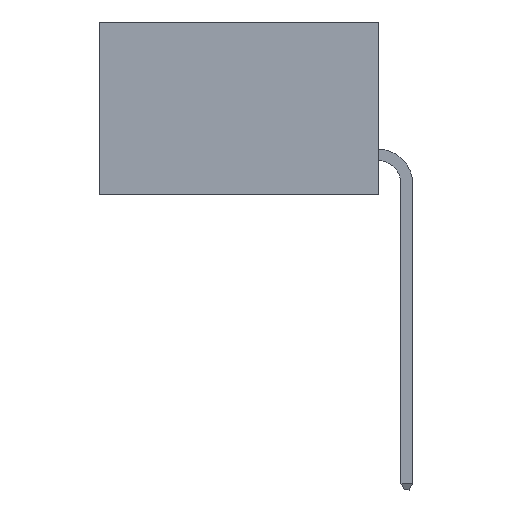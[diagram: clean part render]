
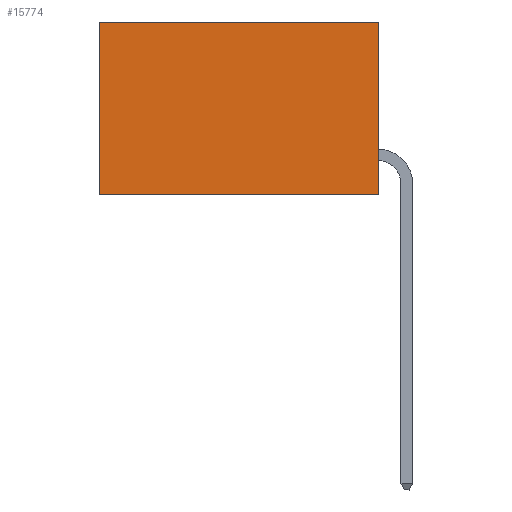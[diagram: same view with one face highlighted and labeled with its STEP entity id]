
A CAD part, left-side view. The second image highlights one B-rep face of the part: STEP entity #15774.
In plain terms, the highlighted planar face has unit normal (-1, 0, 0).
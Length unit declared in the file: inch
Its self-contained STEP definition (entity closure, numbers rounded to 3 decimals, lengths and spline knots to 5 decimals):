
#78 = ORIENTED_EDGE ( 'NONE', *, *, #14140, .T. ) ;
#652 = CARTESIAN_POINT ( 'NONE',  ( 0.298, 0., 0. ) ) ;
#923 = ORIENTED_EDGE ( 'NONE', *, *, #11105, .F. ) ;
#1417 = VERTEX_POINT ( 'NONE', #21766 ) ;
#1817 = LINE ( 'NONE', #8845, #7195 ) ;
#3545 = PLANE ( 'NONE',  #12620 ) ;
#3612 = VERTEX_POINT ( 'NONE', #7756 ) ;
#3830 = VECTOR ( 'NONE', #17193, 39.37008 ) ;
#5278 = ORIENTED_EDGE ( 'NONE', *, *, #18916, .F. ) ;
#5939 = EDGE_LOOP ( 'NONE', ( #15491, #5278, #923, #78 ) ) ;
#6220 = VECTOR ( 'NONE', #10168, 39.37008 ) ;
#6861 = LINE ( 'NONE', #8173, #6220 ) ;
#7195 = VECTOR ( 'NONE', #18887, 39.37008 ) ;
#7619 = DIRECTION ( 'NONE',  ( 1., 0., 0. ) ) ;
#7756 = CARTESIAN_POINT ( 'NONE',  ( 0.298, 0., -0.37 ) ) ;
#8173 = CARTESIAN_POINT ( 'NONE',  ( 0.298, 0.6, 0. ) ) ;
#8714 = VECTOR ( 'NONE', #22568, 39.37008 ) ;
#8845 = CARTESIAN_POINT ( 'NONE',  ( 0.298, 0., -0.37 ) ) ;
#9205 = LINE ( 'NONE', #19108, #3830 ) ;
#10168 = DIRECTION ( 'NONE',  ( 0., 0., -1. ) ) ;
#10492 = FACE_OUTER_BOUND ( 'NONE', #5939, .T. ) ;
#11105 = EDGE_CURVE ( 'NONE', #11674, #3612, #9205, .T. ) ;
#11674 = VERTEX_POINT ( 'NONE', #652 ) ;
#12620 = AXIS2_PLACEMENT_3D ( 'NONE', #25580, #7619, #21693 ) ;
#14073 = LINE ( 'NONE', #20533, #8714 ) ;
#14140 = EDGE_CURVE ( 'NONE', #11674, #1417, #14073, .T. ) ;
#15414 = CARTESIAN_POINT ( 'NONE',  ( 0.298, 0.6, -0.37 ) ) ;
#15491 = ORIENTED_EDGE ( 'NONE', *, *, #20212, .T. ) ;
#15774 = ADVANCED_FACE ( 'NONE', ( #10492 ), #3545, .F. ) ;
#17193 = DIRECTION ( 'NONE',  ( 0., 0., -1. ) ) ;
#18887 = DIRECTION ( 'NONE',  ( 0., 1., 0. ) ) ;
#18916 = EDGE_CURVE ( 'NONE', #3612, #24660, #1817, .T. ) ;
#19108 = CARTESIAN_POINT ( 'NONE',  ( 0.298, 0., 0. ) ) ;
#20212 = EDGE_CURVE ( 'NONE', #1417, #24660, #6861, .T. ) ;
#20533 = CARTESIAN_POINT ( 'NONE',  ( 0.298, 0., 0. ) ) ;
#21693 = DIRECTION ( 'NONE',  ( 0., 0., -1. ) ) ;
#21766 = CARTESIAN_POINT ( 'NONE',  ( 0.298, 0.6, 0. ) ) ;
#22568 = DIRECTION ( 'NONE',  ( 0., 1., 0. ) ) ;
#24660 = VERTEX_POINT ( 'NONE', #15414 ) ;
#25580 = CARTESIAN_POINT ( 'NONE',  ( 0.298, 0., 0. ) ) ;
